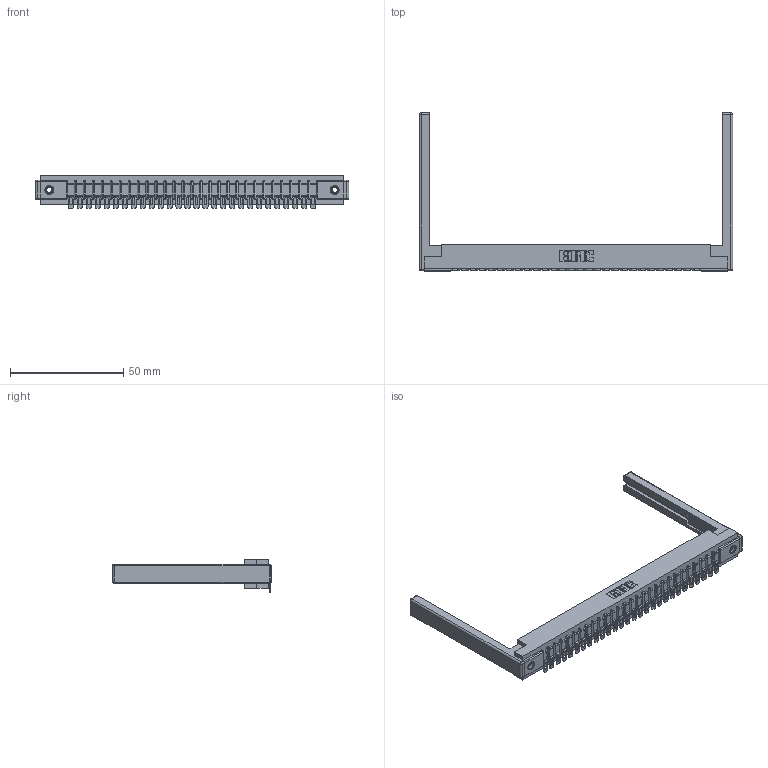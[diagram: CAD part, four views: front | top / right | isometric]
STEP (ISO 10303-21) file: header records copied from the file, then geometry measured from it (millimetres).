
FILE_DESCRIPTION (( 'STEP AP203' ), '1' );
FILE_NAME ('357-028-554-168.STEP', '2019-09-17T02:20:26', ( '' ), ( '' ), 'SwSTEP 2.0', 'SolidWorks 2016', '' );
FILE_SCHEMA (( 'CONFIG_CONTROL_DESIGN' ));
Length unit declared in the file: inch
Products named in the file (5): 307-220-068; 307-290-002_554; 307 Part_.156 Dia Mounting Holes; 357-028-554-168; 345-250-001_345-250-001-102
Assembly tree (33 placements, depth 2):
  357-028-554-168
    307 Part_.156 Dia Mounting Holes
    307-290-002_554  x28
    307-220-068  x2
    345-250-001_345-250-001-102  x2
Bounding box: 138.38 x 69.98 x 14.52 mm (x, y, z)
Volume: 19091.6 mm3; surface area: 22263.3 mm2
Topology: 33 solids, 33 shells, 2569 faces, 7797 edges, 5098 vertices
Faces by surface type: plane 1446, cylinder 1041, sphere 66, cone 12, torus 4
Entity records: 29454 total; most frequent: CARTESIAN_POINT 4931, ORIENTED_EDGE 4910, DIRECTION 4821, EDGE_CURVE 2455, VECTOR 1865, LINE 1865, VERTEX_POINT 1588, AXIS2_PLACEMENT_3D 1478
